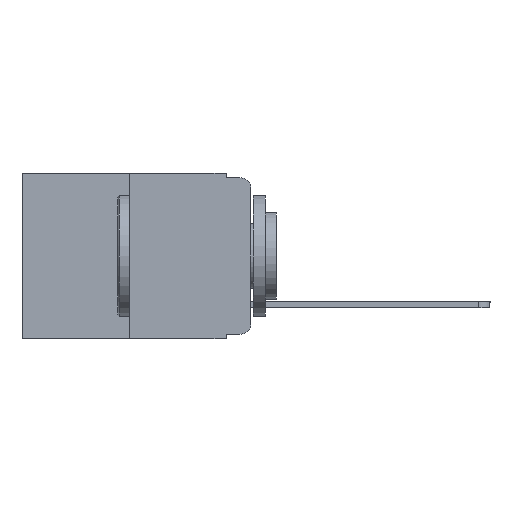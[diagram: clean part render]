
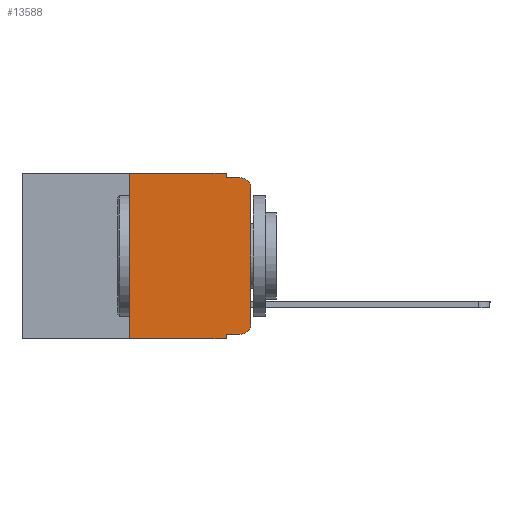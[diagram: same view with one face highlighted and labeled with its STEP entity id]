
A CAD part, left-side view. The second image highlights one B-rep face of the part: STEP entity #13588.
In plain terms, the highlighted planar face has unit normal (-1, 0, 0).
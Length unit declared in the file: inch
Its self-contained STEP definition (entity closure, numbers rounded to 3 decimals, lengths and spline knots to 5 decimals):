
#301 = EDGE_CURVE ( 'NONE', #17348, #1084, #20629, .T. ) ;
#435 = DIRECTION ( 'NONE',  ( -1., 0., 0. ) ) ;
#804 = CIRCLE ( 'NONE', #14707, 0.02 ) ;
#875 = LINE ( 'NONE', #12130, #9960 ) ;
#877 = CARTESIAN_POINT ( 'NONE',  ( 0., 0.051, 0. ) ) ;
#1053 = DIRECTION ( 'NONE',  ( 0., -1., 0. ) ) ;
#1084 = VERTEX_POINT ( 'NONE', #18348 ) ;
#1253 = LINE ( 'NONE', #15984, #3072 ) ;
#1510 = ORIENTED_EDGE ( 'NONE', *, *, #6078, .T. ) ;
#3072 = VECTOR ( 'NONE', #14304, 39.37008 ) ;
#3330 = DIRECTION ( 'NONE',  ( 1., 0., 0. ) ) ;
#3434 = VERTEX_POINT ( 'NONE', #7268 ) ;
#3718 = VERTEX_POINT ( 'NONE', #6610 ) ;
#3720 = VECTOR ( 'NONE', #8139, 39.37008 ) ;
#3989 = VERTEX_POINT ( 'NONE', #17681 ) ;
#4016 = CARTESIAN_POINT ( 'NONE',  ( 0., 0.051, 0. ) ) ;
#4259 = ORIENTED_EDGE ( 'NONE', *, *, #301, .F. ) ;
#4426 = AXIS2_PLACEMENT_3D ( 'NONE', #16311, #16113, #6455 ) ;
#4929 = LINE ( 'NONE', #877, #7573 ) ;
#5084 = DIRECTION ( 'NONE',  ( 0., 0., -1. ) ) ;
#5625 = VERTEX_POINT ( 'NONE', #18944 ) ;
#6078 = EDGE_CURVE ( 'NONE', #19479, #5625, #17942, .T. ) ;
#6132 = EDGE_CURVE ( 'NONE', #3718, #3989, #17843, .T. ) ;
#6455 = DIRECTION ( 'NONE',  ( 0., 0., -1. ) ) ;
#6478 = CARTESIAN_POINT ( 'NONE',  ( 0., 0.02, -0.03 ) ) ;
#6610 = CARTESIAN_POINT ( 'NONE',  ( 0., 0.25, -0.343 ) ) ;
#6677 = EDGE_LOOP ( 'NONE', ( #1510, #20491, #4259, #11122, #19642, #15594, #12295, #15464, #13988, #16073 ) ) ;
#7160 = EDGE_CURVE ( 'NONE', #3434, #19479, #13246, .T. ) ;
#7268 = CARTESIAN_POINT ( 'NONE',  ( 0., 0.02, -0.333 ) ) ;
#7349 = DIRECTION ( 'NONE',  ( 0., 0., -1. ) ) ;
#7471 = VECTOR ( 'NONE', #9908, 39.37008 ) ;
#7573 = VECTOR ( 'NONE', #7349, 39.37008 ) ;
#8139 = DIRECTION ( 'NONE',  ( 0., -1., 0. ) ) ;
#8630 = DIRECTION ( 'NONE',  ( 0., 0., 1. ) ) ;
#9908 = DIRECTION ( 'NONE',  ( 0., 0., 1. ) ) ;
#9960 = VECTOR ( 'NONE', #18456, 39.37008 ) ;
#10116 = CARTESIAN_POINT ( 'NONE',  ( 0., 0.25, 0. ) ) ;
#11102 = EDGE_CURVE ( 'NONE', #14932, #17348, #17803, .T. ) ;
#11122 = ORIENTED_EDGE ( 'NONE', *, *, #11102, .F. ) ;
#11704 = DIRECTION ( 'NONE',  ( 0., 0., -1. ) ) ;
#11823 = VERTEX_POINT ( 'NONE', #20697 ) ;
#12130 = CARTESIAN_POINT ( 'NONE',  ( 0., 0.473, -0.343 ) ) ;
#12243 = CARTESIAN_POINT ( 'NONE',  ( 0., 0.051, -0.333 ) ) ;
#12295 = ORIENTED_EDGE ( 'NONE', *, *, #19237, .T. ) ;
#13057 = CARTESIAN_POINT ( 'NONE',  ( 0., 0.051, 0. ) ) ;
#13076 = DIRECTION ( 'NONE',  ( 0., 0., -1. ) ) ;
#13246 = CIRCLE ( 'NONE', #4426, 0.02 ) ;
#13588 = ADVANCED_FACE ( 'NONE', ( #16352 ), #19514, .F. ) ;
#13988 = ORIENTED_EDGE ( 'NONE', *, *, #15176, .T. ) ;
#14101 = CARTESIAN_POINT ( 'NONE',  ( 0., 0.051, -0.01 ) ) ;
#14304 = DIRECTION ( 'NONE',  ( 0., -1., 0. ) ) ;
#14707 = AXIS2_PLACEMENT_3D ( 'NONE', #6478, #435, #13076 ) ;
#14813 = VECTOR ( 'NONE', #1053, 39.37008 ) ;
#14932 = VERTEX_POINT ( 'NONE', #4016 ) ;
#15176 = EDGE_CURVE ( 'NONE', #16060, #3434, #19557, .T. ) ;
#15464 = ORIENTED_EDGE ( 'NONE', *, *, #20459, .F. ) ;
#15594 = ORIENTED_EDGE ( 'NONE', *, *, #6132, .F. ) ;
#15604 = VECTOR ( 'NONE', #8630, 39.37008 ) ;
#15833 = CARTESIAN_POINT ( 'NONE',  ( 0., 0.051, -0.01 ) ) ;
#15984 = CARTESIAN_POINT ( 'NONE',  ( 0., 0.473, 0. ) ) ;
#16060 = VERTEX_POINT ( 'NONE', #12243 ) ;
#16073 = ORIENTED_EDGE ( 'NONE', *, *, #7160, .T. ) ;
#16113 = DIRECTION ( 'NONE',  ( -1., 0., 0. ) ) ;
#16258 = CARTESIAN_POINT ( 'NONE',  ( 0., 0., 0. ) ) ;
#16289 = CARTESIAN_POINT ( 'NONE',  ( 0., 0.051, -0.333 ) ) ;
#16311 = CARTESIAN_POINT ( 'NONE',  ( 0., 0.02, -0.313 ) ) ;
#16352 = FACE_OUTER_BOUND ( 'NONE', #6677, .T. ) ;
#16414 = EDGE_CURVE ( 'NONE', #3989, #14932, #1253, .T. ) ;
#17348 = VERTEX_POINT ( 'NONE', #15833 ) ;
#17681 = CARTESIAN_POINT ( 'NONE',  ( 0., 0.25, 0. ) ) ;
#17803 = LINE ( 'NONE', #13057, #20110 ) ;
#17843 = LINE ( 'NONE', #10116, #15604 ) ;
#17942 = LINE ( 'NONE', #16258, #7471 ) ;
#18348 = CARTESIAN_POINT ( 'NONE',  ( 0., 0.02, -0.01 ) ) ;
#18456 = DIRECTION ( 'NONE',  ( 0., -1., 0. ) ) ;
#18944 = CARTESIAN_POINT ( 'NONE',  ( 0., 0., -0.03 ) ) ;
#19237 = EDGE_CURVE ( 'NONE', #3718, #11823, #875, .T. ) ;
#19411 = CARTESIAN_POINT ( 'NONE',  ( 0., 0.473, 0. ) ) ;
#19479 = VERTEX_POINT ( 'NONE', #20657 ) ;
#19514 = PLANE ( 'NONE',  #20464 ) ;
#19557 = LINE ( 'NONE', #16289, #3720 ) ;
#19642 = ORIENTED_EDGE ( 'NONE', *, *, #16414, .F. ) ;
#20110 = VECTOR ( 'NONE', #5084, 39.37008 ) ;
#20459 = EDGE_CURVE ( 'NONE', #16060, #11823, #4929, .T. ) ;
#20464 = AXIS2_PLACEMENT_3D ( 'NONE', #19411, #3330, #11704 ) ;
#20491 = ORIENTED_EDGE ( 'NONE', *, *, #20772, .T. ) ;
#20629 = LINE ( 'NONE', #14101, #14813 ) ;
#20657 = CARTESIAN_POINT ( 'NONE',  ( 0., 0., -0.313 ) ) ;
#20697 = CARTESIAN_POINT ( 'NONE',  ( 0., 0.051, -0.343 ) ) ;
#20772 = EDGE_CURVE ( 'NONE', #5625, #1084, #804, .T. ) ;
